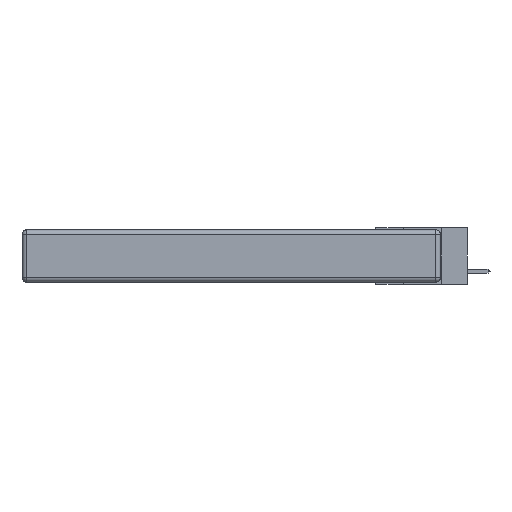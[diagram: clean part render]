
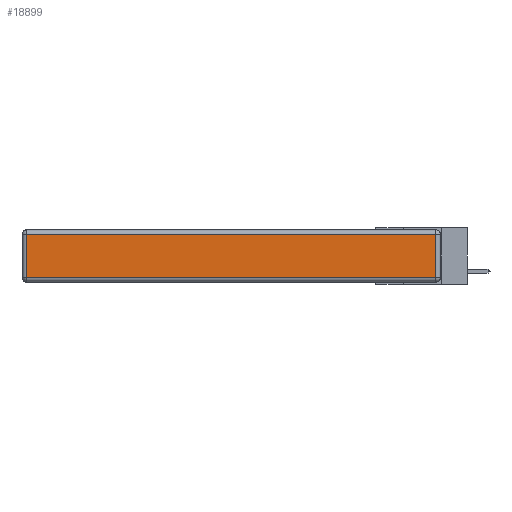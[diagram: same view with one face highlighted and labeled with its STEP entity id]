
A CAD part, left-side view. The second image highlights one B-rep face of the part: STEP entity #18899.
In plain terms, the highlighted planar face has unit normal (-1, 0, 0).
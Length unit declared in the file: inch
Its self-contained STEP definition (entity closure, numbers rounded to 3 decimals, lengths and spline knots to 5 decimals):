
#201 = ORIENTED_EDGE ( 'NONE', *, *, #6313, .T. ) ;
#1702 = LINE ( 'NONE', #15279, #21299 ) ;
#2025 = DIRECTION ( 'NONE',  ( 0., 0., 1. ) ) ;
#2298 = ORIENTED_EDGE ( 'NONE', *, *, #15291, .T. ) ;
#2442 = CARTESIAN_POINT ( 'NONE',  ( 0., 2.72, -0.313 ) ) ;
#2662 = VECTOR ( 'NONE', #11956, 39.37008 ) ;
#3273 = VECTOR ( 'NONE', #19504, 39.37008 ) ;
#4338 = CARTESIAN_POINT ( 'NONE',  ( 0., 0., -0.343 ) ) ;
#4989 = EDGE_CURVE ( 'NONE', #17488, #17329, #15301, .T. ) ;
#5698 = EDGE_CURVE ( 'NONE', #17329, #10781, #7374, .T. ) ;
#6313 = EDGE_CURVE ( 'NONE', #10781, #15289, #22848, .T. ) ;
#7374 = LINE ( 'NONE', #17984, #3273 ) ;
#8605 = DIRECTION ( 'NONE',  ( 0., 1., 0. ) ) ;
#10635 = AXIS2_PLACEMENT_3D ( 'NONE', #4338, #21024, #15375 ) ;
#10781 = VERTEX_POINT ( 'NONE', #2442 ) ;
#11956 = DIRECTION ( 'NONE',  ( 0., -1., 0. ) ) ;
#12555 = ORIENTED_EDGE ( 'NONE', *, *, #4989, .T. ) ;
#12832 = FACE_OUTER_BOUND ( 'NONE', #20847, .T. ) ;
#14196 = ORIENTED_EDGE ( 'NONE', *, *, #5698, .T. ) ;
#15279 = CARTESIAN_POINT ( 'NONE',  ( 0., 0.03, -0.343 ) ) ;
#15289 = VERTEX_POINT ( 'NONE', #20604 ) ;
#15291 = EDGE_CURVE ( 'NONE', #15289, #17488, #1702, .T. ) ;
#15301 = LINE ( 'NONE', #17887, #22921 ) ;
#15375 = DIRECTION ( 'NONE',  ( 0., 0., 1. ) ) ;
#16714 = CARTESIAN_POINT ( 'NONE',  ( 0., 2.72, -0.03 ) ) ;
#16785 = CARTESIAN_POINT ( 'NONE',  ( 0., 0.03, -0.03 ) ) ;
#17329 = VERTEX_POINT ( 'NONE', #16714 ) ;
#17488 = VERTEX_POINT ( 'NONE', #16785 ) ;
#17887 = CARTESIAN_POINT ( 'NONE',  ( 0., 2.75, -0.03 ) ) ;
#17984 = CARTESIAN_POINT ( 'NONE',  ( 0., 2.72, -0.343 ) ) ;
#18899 = ADVANCED_FACE ( 'NONE', ( #12832 ), #22843, .T. ) ;
#19504 = DIRECTION ( 'NONE',  ( 0., 0., -1. ) ) ;
#20604 = CARTESIAN_POINT ( 'NONE',  ( 0., 0.03, -0.313 ) ) ;
#20847 = EDGE_LOOP ( 'NONE', ( #201, #2298, #12555, #14196 ) ) ;
#21024 = DIRECTION ( 'NONE',  ( -1., 0., 0. ) ) ;
#21299 = VECTOR ( 'NONE', #2025, 39.37008 ) ;
#22843 = PLANE ( 'NONE',  #10635 ) ;
#22848 = LINE ( 'NONE', #23257, #2662 ) ;
#22921 = VECTOR ( 'NONE', #8605, 39.37008 ) ;
#23257 = CARTESIAN_POINT ( 'NONE',  ( 0., 0., -0.313 ) ) ;
